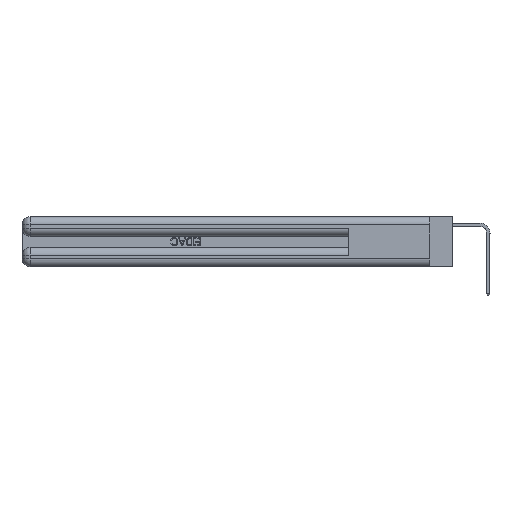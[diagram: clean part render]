
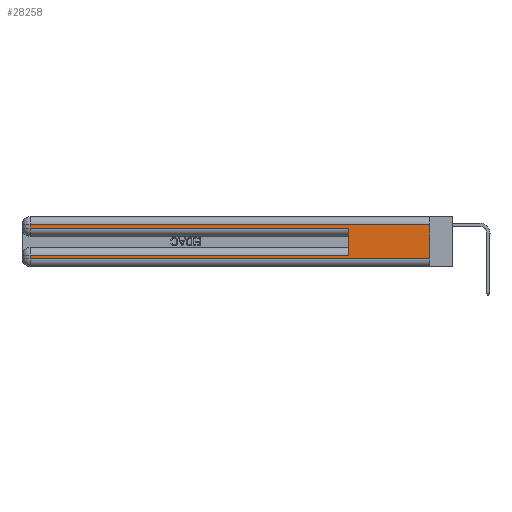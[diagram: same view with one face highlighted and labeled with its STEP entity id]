
A CAD part, left-side view. The second image highlights one B-rep face of the part: STEP entity #28258.
In plain terms, the highlighted planar face has unit normal (-1, 0, 0).
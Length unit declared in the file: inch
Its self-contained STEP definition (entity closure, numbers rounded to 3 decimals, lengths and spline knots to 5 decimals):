
#541 = LINE ( 'NONE', #19076, #28079 ) ;
#880 = DIRECTION ( 'NONE',  ( 0., -1., 0. ) ) ;
#1131 = EDGE_CURVE ( 'NONE', #32058, #6359, #20858, .T. ) ;
#1162 = VECTOR ( 'NONE', #5128, 39.37008 ) ;
#1186 = LINE ( 'NONE', #18248, #9026 ) ;
#1222 = EDGE_CURVE ( 'NONE', #22076, #18579, #11636, .T. ) ;
#1367 = ORIENTED_EDGE ( 'NONE', *, *, #1131, .F. ) ;
#1711 = VECTOR ( 'NONE', #3373, 39.37008 ) ;
#2113 = CARTESIAN_POINT ( 'NONE',  ( 0., 0.6, 0.145 ) ) ;
#2457 = CARTESIAN_POINT ( 'NONE',  ( 0., 0., 0.37 ) ) ;
#2562 = DIRECTION ( 'NONE',  ( 1., 0., 0. ) ) ;
#2701 = DIRECTION ( 'NONE',  ( 0., 1., 0. ) ) ;
#3373 = DIRECTION ( 'NONE',  ( 0., -1., 0. ) ) ;
#3572 = ORIENTED_EDGE ( 'NONE', *, *, #1222, .T. ) ;
#4020 = ORIENTED_EDGE ( 'NONE', *, *, #30371, .F. ) ;
#4863 = CARTESIAN_POINT ( 'NONE',  ( 0., 0., 0.31 ) ) ;
#5128 = DIRECTION ( 'NONE',  ( 0., 0., -1. ) ) ;
#6359 = VERTEX_POINT ( 'NONE', #19063 ) ;
#6447 = EDGE_LOOP ( 'NONE', ( #4020, #23741, #3572, #14538, #1367, #32957, #28013, #27498 ) ) ;
#7004 = EDGE_CURVE ( 'NONE', #8016, #28528, #18969, .T. ) ;
#7138 = VECTOR ( 'NONE', #17684, 39.37008 ) ;
#7382 = LINE ( 'NONE', #31114, #21919 ) ;
#7423 = CARTESIAN_POINT ( 'NONE',  ( 0., 0.6, 0.085 ) ) ;
#7632 = DIRECTION ( 'NONE',  ( 0., 0., -1. ) ) ;
#7965 = VERTEX_POINT ( 'NONE', #12513 ) ;
#8016 = VERTEX_POINT ( 'NONE', #30601 ) ;
#8344 = EDGE_CURVE ( 'NONE', #18579, #6359, #541, .T. ) ;
#9026 = VECTOR ( 'NONE', #2701, 39.37008 ) ;
#9442 = EDGE_CURVE ( 'NONE', #28528, #7965, #22429, .T. ) ;
#11122 = EDGE_CURVE ( 'NONE', #32058, #8016, #7382, .T. ) ;
#11356 = VECTOR ( 'NONE', #14462, 39.37008 ) ;
#11636 = LINE ( 'NONE', #25612, #12446 ) ;
#11765 = EDGE_CURVE ( 'NONE', #30819, #22076, #1186, .T. ) ;
#12446 = VECTOR ( 'NONE', #7632, 39.37008 ) ;
#12513 = CARTESIAN_POINT ( 'NONE',  ( 0., 0., 0.06 ) ) ;
#14462 = DIRECTION ( 'NONE',  ( 0., 0., -1. ) ) ;
#14538 = ORIENTED_EDGE ( 'NONE', *, *, #8344, .T. ) ;
#17684 = DIRECTION ( 'NONE',  ( 0., 0., 1. ) ) ;
#18120 = CARTESIAN_POINT ( 'NONE',  ( 0., 0., 0.37 ) ) ;
#18248 = CARTESIAN_POINT ( 'NONE',  ( 0., 0., 0.31 ) ) ;
#18579 = VERTEX_POINT ( 'NONE', #22903 ) ;
#18903 = CARTESIAN_POINT ( 'NONE',  ( 0., 0., 0.06 ) ) ;
#18969 = LINE ( 'NONE', #32290, #11356 ) ;
#19063 = CARTESIAN_POINT ( 'NONE',  ( 0., 0.6, 0.285 ) ) ;
#19076 = CARTESIAN_POINT ( 'NONE',  ( 0., 0., 0.285 ) ) ;
#20502 = CARTESIAN_POINT ( 'NONE',  ( 0., 2.94, 0.31 ) ) ;
#20700 = DIRECTION ( 'NONE',  ( 0., 0., -1. ) ) ;
#20858 = LINE ( 'NONE', #2113, #7138 ) ;
#21919 = VECTOR ( 'NONE', #28679, 39.37008 ) ;
#22076 = VERTEX_POINT ( 'NONE', #20502 ) ;
#22109 = AXIS2_PLACEMENT_3D ( 'NONE', #18120, #2562, #20700 ) ;
#22429 = LINE ( 'NONE', #18903, #1711 ) ;
#22701 = LINE ( 'NONE', #2457, #1162 ) ;
#22903 = CARTESIAN_POINT ( 'NONE',  ( 0., 2.94, 0.285 ) ) ;
#23741 = ORIENTED_EDGE ( 'NONE', *, *, #11765, .T. ) ;
#25612 = CARTESIAN_POINT ( 'NONE',  ( 0., 2.94, 0.37 ) ) ;
#27498 = ORIENTED_EDGE ( 'NONE', *, *, #9442, .T. ) ;
#28013 = ORIENTED_EDGE ( 'NONE', *, *, #7004, .T. ) ;
#28079 = VECTOR ( 'NONE', #880, 39.37008 ) ;
#28258 = ADVANCED_FACE ( 'NONE', ( #30031 ), #33170, .F. ) ;
#28528 = VERTEX_POINT ( 'NONE', #31836 ) ;
#28679 = DIRECTION ( 'NONE',  ( 0., 1., 0. ) ) ;
#30031 = FACE_OUTER_BOUND ( 'NONE', #6447, .T. ) ;
#30371 = EDGE_CURVE ( 'NONE', #30819, #7965, #22701, .T. ) ;
#30601 = CARTESIAN_POINT ( 'NONE',  ( 0., 2.94, 0.085 ) ) ;
#30819 = VERTEX_POINT ( 'NONE', #4863 ) ;
#31114 = CARTESIAN_POINT ( 'NONE',  ( 0., 0., 0.085 ) ) ;
#31836 = CARTESIAN_POINT ( 'NONE',  ( 0., 2.94, 0.06 ) ) ;
#32058 = VERTEX_POINT ( 'NONE', #7423 ) ;
#32290 = CARTESIAN_POINT ( 'NONE',  ( 0., 2.94, 0.37 ) ) ;
#32957 = ORIENTED_EDGE ( 'NONE', *, *, #11122, .T. ) ;
#33170 = PLANE ( 'NONE',  #22109 ) ;
